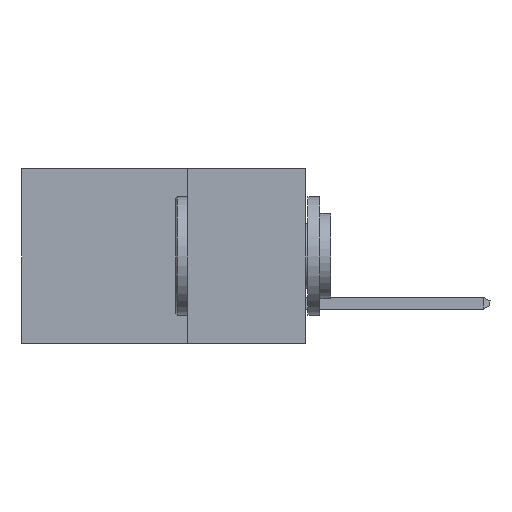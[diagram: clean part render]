
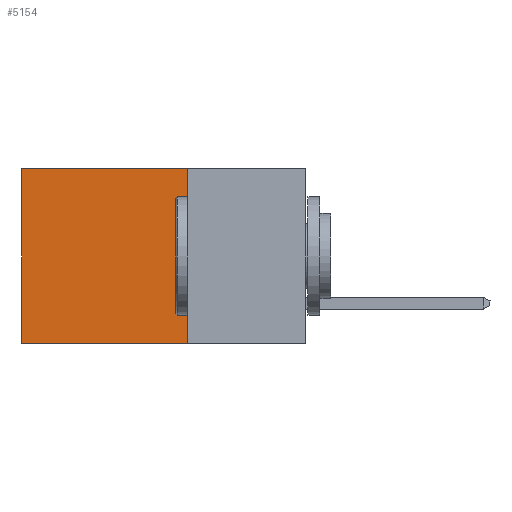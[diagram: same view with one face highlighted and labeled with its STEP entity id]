
A CAD part, left-side view. The second image highlights one B-rep face of the part: STEP entity #5154.
In plain terms, the highlighted planar face has unit normal (-1, 0, 0).
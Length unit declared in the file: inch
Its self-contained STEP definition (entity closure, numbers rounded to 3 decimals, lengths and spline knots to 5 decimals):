
#693 = ORIENTED_EDGE ( 'NONE', *, *, #15041, .T. ) ;
#1391 = LINE ( 'NONE', #16465, #9615 ) ;
#2231 = LINE ( 'NONE', #20454, #20580 ) ;
#2647 = CARTESIAN_POINT ( 'NONE',  ( 0.2615, 0.6, -0.37 ) ) ;
#3292 = EDGE_CURVE ( 'NONE', #26767, #21129, #8001, .T. ) ;
#3851 = VECTOR ( 'NONE', #6217, 39.37008 ) ;
#5154 = ADVANCED_FACE ( 'NONE', ( #13378 ), #25346, .F. ) ;
#6016 = AXIS2_PLACEMENT_3D ( 'NONE', #23436, #23701, #15433 ) ;
#6217 = DIRECTION ( 'NONE',  ( 0., 0., -1. ) ) ;
#8001 = LINE ( 'NONE', #14775, #3851 ) ;
#8341 = ORIENTED_EDGE ( 'NONE', *, *, #20162, .F. ) ;
#8473 = VECTOR ( 'NONE', #10532, 39.37008 ) ;
#9615 = VECTOR ( 'NONE', #22169, 39.37008 ) ;
#10532 = DIRECTION ( 'NONE',  ( 0., 0., -1. ) ) ;
#12580 = LINE ( 'NONE', #25085, #8473 ) ;
#13378 = FACE_OUTER_BOUND ( 'NONE', #22951, .T. ) ;
#13830 = VERTEX_POINT ( 'NONE', #14989 ) ;
#14775 = CARTESIAN_POINT ( 'NONE',  ( 0.2615, 0.25, -0.37 ) ) ;
#14989 = CARTESIAN_POINT ( 'NONE',  ( 0.2615, 0.6, 0. ) ) ;
#15041 = EDGE_CURVE ( 'NONE', #13830, #15191, #12580, .T. ) ;
#15191 = VERTEX_POINT ( 'NONE', #2647 ) ;
#15433 = DIRECTION ( 'NONE',  ( 0., 0., -1. ) ) ;
#16263 = CARTESIAN_POINT ( 'NONE',  ( 0.2615, 0.25, 0. ) ) ;
#16387 = DIRECTION ( 'NONE',  ( 0., 1., 0. ) ) ;
#16465 = CARTESIAN_POINT ( 'NONE',  ( 0.2615, 0.25, -0.37 ) ) ;
#16621 = ORIENTED_EDGE ( 'NONE', *, *, #3292, .F. ) ;
#16651 = ORIENTED_EDGE ( 'NONE', *, *, #25434, .T. ) ;
#20162 = EDGE_CURVE ( 'NONE', #21129, #15191, #1391, .T. ) ;
#20454 = CARTESIAN_POINT ( 'NONE',  ( 0.2615, 0.25, 0. ) ) ;
#20580 = VECTOR ( 'NONE', #16387, 39.37008 ) ;
#21129 = VERTEX_POINT ( 'NONE', #21239 ) ;
#21239 = CARTESIAN_POINT ( 'NONE',  ( 0.2615, 0.25, -0.37 ) ) ;
#22169 = DIRECTION ( 'NONE',  ( 0., 1., 0. ) ) ;
#22951 = EDGE_LOOP ( 'NONE', ( #693, #8341, #16621, #16651 ) ) ;
#23436 = CARTESIAN_POINT ( 'NONE',  ( 0.2615, 0.25, -0.37 ) ) ;
#23701 = DIRECTION ( 'NONE',  ( 1., 0., 0. ) ) ;
#25085 = CARTESIAN_POINT ( 'NONE',  ( 0.2615, 0.6, -0.37 ) ) ;
#25346 = PLANE ( 'NONE',  #6016 ) ;
#25434 = EDGE_CURVE ( 'NONE', #26767, #13830, #2231, .T. ) ;
#26767 = VERTEX_POINT ( 'NONE', #16263 ) ;
